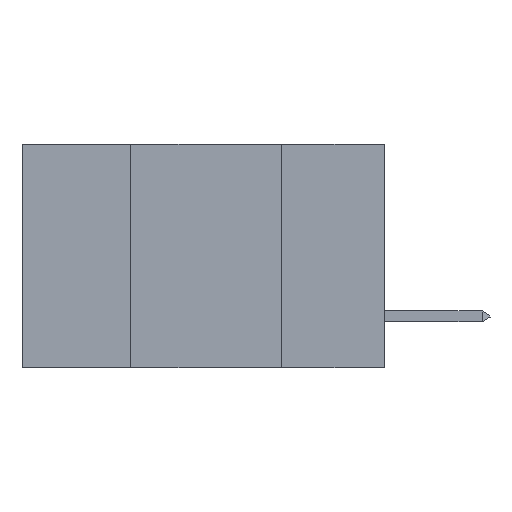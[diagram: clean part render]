
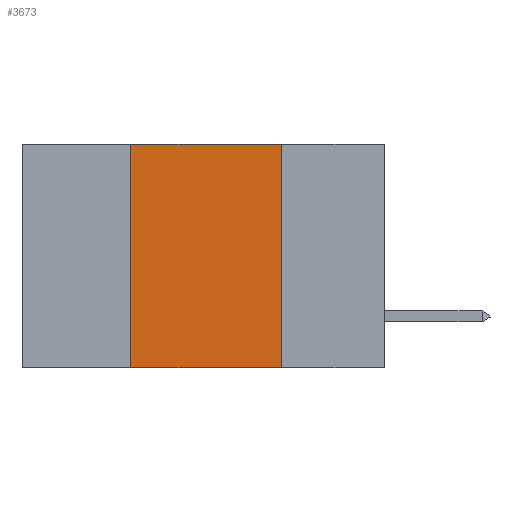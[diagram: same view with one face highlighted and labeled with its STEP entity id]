
A CAD part, left-side view. The second image highlights one B-rep face of the part: STEP entity #3673.
In plain terms, the highlighted planar face has unit normal (-1, 0, 0).
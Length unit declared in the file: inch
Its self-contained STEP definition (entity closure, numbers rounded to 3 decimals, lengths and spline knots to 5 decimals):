
#210 = DIRECTION ( 'NONE',  ( 0., -1., 0. ) ) ;
#745 = FACE_OUTER_BOUND ( 'NONE', #14624, .T. ) ;
#3084 = ORIENTED_EDGE ( 'NONE', *, *, #10432, .T. ) ;
#3673 = ADVANCED_FACE ( 'NONE', ( #745 ), #7583, .F. ) ;
#4165 = EDGE_CURVE ( 'NONE', #16854, #13761, #21164, .T. ) ;
#4191 = DIRECTION ( 'NONE',  ( 0., -1., 0. ) ) ;
#4948 = LINE ( 'NONE', #8915, #5185 ) ;
#5185 = VECTOR ( 'NONE', #10384, 39.37008 ) ;
#5278 = CARTESIAN_POINT ( 'NONE',  ( 0., 0.42, 0. ) ) ;
#5919 = DIRECTION ( 'NONE',  ( 0., 0., -1. ) ) ;
#7443 = DIRECTION ( 'NONE',  ( 1., 0., 0. ) ) ;
#7583 = PLANE ( 'NONE',  #16137 ) ;
#8250 = ORIENTED_EDGE ( 'NONE', *, *, #11694, .F. ) ;
#8705 = CARTESIAN_POINT ( 'NONE',  ( 0., 0.6, 0. ) ) ;
#8915 = CARTESIAN_POINT ( 'NONE',  ( 0., 0.42, 0. ) ) ;
#8988 = LINE ( 'NONE', #8705, #14843 ) ;
#9196 = ORIENTED_EDGE ( 'NONE', *, *, #4165, .F. ) ;
#9493 = VERTEX_POINT ( 'NONE', #5278 ) ;
#10294 = VECTOR ( 'NONE', #4191, 39.37008 ) ;
#10384 = DIRECTION ( 'NONE',  ( 0., 0., 1. ) ) ;
#10432 = EDGE_CURVE ( 'NONE', #12400, #13761, #15075, .T. ) ;
#11694 = EDGE_CURVE ( 'NONE', #9493, #16854, #8988, .T. ) ;
#12400 = VERTEX_POINT ( 'NONE', #18199 ) ;
#13761 = VERTEX_POINT ( 'NONE', #14204 ) ;
#14204 = CARTESIAN_POINT ( 'NONE',  ( 0., 0.17, -0.37 ) ) ;
#14624 = EDGE_LOOP ( 'NONE', ( #9196, #8250, #20706, #3084 ) ) ;
#14843 = VECTOR ( 'NONE', #210, 39.37008 ) ;
#15075 = LINE ( 'NONE', #20789, #10294 ) ;
#16071 = CARTESIAN_POINT ( 'NONE',  ( 0., 0.17, 0. ) ) ;
#16137 = AXIS2_PLACEMENT_3D ( 'NONE', #21092, #7443, #5919 ) ;
#16854 = VERTEX_POINT ( 'NONE', #16071 ) ;
#17476 = VECTOR ( 'NONE', #19823, 39.37008 ) ;
#18199 = CARTESIAN_POINT ( 'NONE',  ( 0., 0.42, -0.37 ) ) ;
#18501 = CARTESIAN_POINT ( 'NONE',  ( 0., 0.17, 0. ) ) ;
#18773 = EDGE_CURVE ( 'NONE', #12400, #9493, #4948, .T. ) ;
#19823 = DIRECTION ( 'NONE',  ( 0., 0., -1. ) ) ;
#20706 = ORIENTED_EDGE ( 'NONE', *, *, #18773, .F. ) ;
#20789 = CARTESIAN_POINT ( 'NONE',  ( 0., 0.6, -0.37 ) ) ;
#21092 = CARTESIAN_POINT ( 'NONE',  ( 0., 0.6, 0. ) ) ;
#21164 = LINE ( 'NONE', #18501, #17476 ) ;
